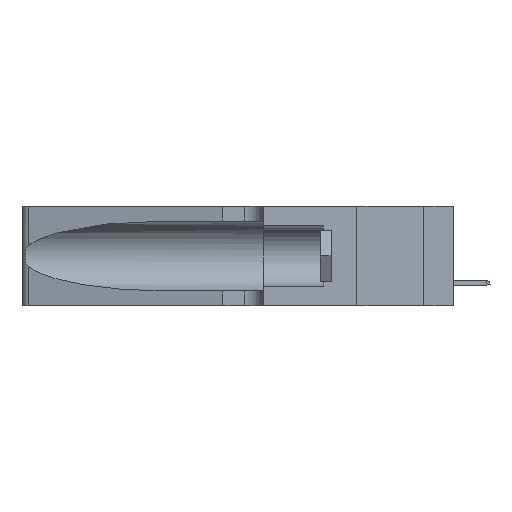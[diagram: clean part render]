
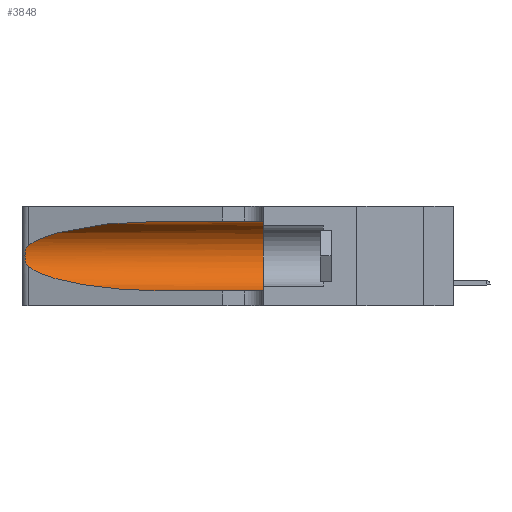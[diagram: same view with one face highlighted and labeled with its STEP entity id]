
A CAD part, left-side view. The second image highlights one B-rep face of the part: STEP entity #3848.
In plain terms, the highlighted cylindrical face has radius 3.308 mm (diameter 6.617 mm), a partial arc.
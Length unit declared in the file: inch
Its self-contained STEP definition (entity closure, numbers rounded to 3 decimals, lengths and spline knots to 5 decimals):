
#426 = EDGE_CURVE ( 'NONE', #11697, #22639, #37055, .T. ) ;
#994 = CARTESIAN_POINT ( 'NONE',  ( 0.25639, 1.23186, 0.15144 ) ) ;
#1021 = ORIENTED_EDGE ( 'NONE', *, *, #30124, .F. ) ;
#1545 = EDGE_CURVE ( 'NONE', #43997, #11697, #33295, .T. ) ;
#1990 = CARTESIAN_POINT ( 'NONE',  ( 0.25854, 1.2359, 0.20912 ) ) ;
#3632 = ORIENTED_EDGE ( 'NONE', *, *, #47640, .T. ) ;
#3848 = ADVANCED_FACE ( 'NONE', ( #8337 ), #12750, .F. ) ;
#4104 = CARTESIAN_POINT ( 'NONE',  ( 0.18966, 0.96281, 0.31525 ) ) ;
#4293 = CARTESIAN_POINT ( 'NONE',  ( 0.1305, 0.35, 0.05475 ) ) ;
#4942 =( BOUNDED_CURVE ( )  B_SPLINE_CURVE ( 3, ( #20145, #4104, #19639, #46591 ),
 .UNSPECIFIED., .F., .F. ) 
 B_SPLINE_CURVE_WITH_KNOTS ( ( 4, 4 ),
 ( 1.5708, 2.84003 ),
 .UNSPECIFIED. ) 
 CURVE ( )  GEOMETRIC_REPRESENTATION_ITEM ( )  RATIONAL_B_SPLINE_CURVE ( ( 1., 0.87, 0.87, 1. ) ) 
 REPRESENTATION_ITEM ( '' )  );
#5125 = CARTESIAN_POINT ( 'NONE',  ( 0.25487, 1.22718, 0.22369 ) ) ;
#5158 = CARTESIAN_POINT ( 'NONE',  ( 0.26018, 1.23835, 0.19895 ) ) ;
#5634 = CARTESIAN_POINT ( 'NONE',  ( 0.25555, 1.22994, 0.2215 ) ) ;
#5789 = CARTESIAN_POINT ( 'NONE',  ( 0.2373, 1.15595, 0.08982 ) ) ;
#6092 = CARTESIAN_POINT ( 'NONE',  ( 0.1305, 0.72297, 0.05475 ) ) ;
#6539 = VECTOR ( 'NONE', #46669, 39.37008 ) ;
#8337 = FACE_OUTER_BOUND ( 'NONE', #47398, .T. ) ;
#8387 = LINE ( 'NONE', #46920, #6539 ) ;
#8390 = CARTESIAN_POINT ( 'NONE',  ( 0.25856, 1.23593, 0.16098 ) ) ;
#11547 = VERTEX_POINT ( 'NONE', #5125 ) ;
#11697 = VERTEX_POINT ( 'NONE', #6092 ) ;
#12750 = CYLINDRICAL_SURFACE ( 'NONE', #36567, 0.13025 ) ;
#12976 = ORIENTED_EDGE ( 'NONE', *, *, #41182, .F. ) ;
#16011 = CARTESIAN_POINT ( 'NONE',  ( 0.25555, 1.22993, 0.14849 ) ) ;
#17529 = VERTEX_POINT ( 'NONE', #19064 ) ;
#19064 = CARTESIAN_POINT ( 'NONE',  ( 0.1305, 0.72297, 0.31525 ) ) ;
#19639 = CARTESIAN_POINT ( 'NONE',  ( 0.2373, 1.15595, 0.28018 ) ) ;
#20145 = CARTESIAN_POINT ( 'NONE',  ( 0.1305, 0.72297, 0.31525 ) ) ;
#21461 = B_SPLINE_CURVE_WITH_KNOTS ( 'NONE', 3,
 ( #28131, #5634, #39008, #35774, #1990, #5158, #30818, #45921, #42231, #8390, #34775, #994, #16011, #31064 ),
 .UNSPECIFIED., .F., .F.,
 ( 4, 2, 2, 2, 2, 2, 4 ),
 ( 0., 0.00027, 0.00053, 0.00107, 0.0016, 0.00187, 0.00214 ),
 .UNSPECIFIED. ) ;
#22549 = CARTESIAN_POINT ( 'NONE',  ( 0.18966, 0.96281, 0.05475 ) ) ;
#22639 = VERTEX_POINT ( 'NONE', #4293 ) ;
#23770 = DIRECTION ( 'NONE',  ( 0., 0., 1. ) ) ;
#23881 = AXIS2_PLACEMENT_3D ( 'NONE', #24027, #46276, #23770 ) ;
#24027 = CARTESIAN_POINT ( 'NONE',  ( 0.1305, 0.35, 0.185 ) ) ;
#24569 = CARTESIAN_POINT ( 'NONE',  ( 0.25487, 1.22718, 0.14631 ) ) ;
#26194 = DIRECTION ( 'NONE',  ( 0., -1., 0. ) ) ;
#27600 = DIRECTION ( 'NONE',  ( 0., -1., 0. ) ) ;
#28053 = EDGE_CURVE ( 'NONE', #17529, #11547, #4942, .T. ) ;
#28131 = CARTESIAN_POINT ( 'NONE',  ( 0.25487, 1.22718, 0.22369 ) ) ;
#29328 = VECTOR ( 'NONE', #26194, 39.37008 ) ;
#30124 = EDGE_CURVE ( 'NONE', #17529, #39484, #8387, .T. ) ;
#30818 = CARTESIAN_POINT ( 'NONE',  ( 0.26075, 1.23896, 0.19203 ) ) ;
#30935 = CIRCLE ( 'NONE', #23881, 0.13025 ) ;
#31064 = CARTESIAN_POINT ( 'NONE',  ( 0.25487, 1.22718, 0.14631 ) ) ;
#33295 =( BOUNDED_CURVE ( )  B_SPLINE_CURVE ( 3, ( #24569, #5789, #22549, #37129 ),
 .UNSPECIFIED., .F., .F. ) 
 B_SPLINE_CURVE_WITH_KNOTS ( ( 4, 4 ),
 ( 3.44316, 4.71239 ),
 .UNSPECIFIED. ) 
 CURVE ( )  GEOMETRIC_REPRESENTATION_ITEM ( )  RATIONAL_B_SPLINE_CURVE ( ( 1., 0.87, 0.87, 1. ) ) 
 REPRESENTATION_ITEM ( '' )  );
#33809 = CARTESIAN_POINT ( 'NONE',  ( 0.1305, 1.61858, 0.05475 ) ) ;
#34775 = CARTESIAN_POINT ( 'NONE',  ( 0.25789, 1.23486, 0.15765 ) ) ;
#35006 = ORIENTED_EDGE ( 'NONE', *, *, #28053, .T. ) ;
#35021 = ORIENTED_EDGE ( 'NONE', *, *, #1545, .T. ) ;
#35774 = CARTESIAN_POINT ( 'NONE',  ( 0.25787, 1.23484, 0.2124 ) ) ;
#36567 = AXIS2_PLACEMENT_3D ( 'NONE', #38219, #27600, #38465 ) ;
#37055 = LINE ( 'NONE', #33809, #29328 ) ;
#37129 = CARTESIAN_POINT ( 'NONE',  ( 0.1305, 0.72297, 0.05475 ) ) ;
#38219 = CARTESIAN_POINT ( 'NONE',  ( 0.1305, 1.61858, 0.185 ) ) ;
#38247 = CARTESIAN_POINT ( 'NONE',  ( 0.1305, 0.35, 0.31525 ) ) ;
#38465 = DIRECTION ( 'NONE',  ( 0., 0., -1. ) ) ;
#39008 = CARTESIAN_POINT ( 'NONE',  ( 0.25639, 1.23184, 0.21858 ) ) ;
#39484 = VERTEX_POINT ( 'NONE', #38247 ) ;
#40387 = CARTESIAN_POINT ( 'NONE',  ( 0.25487, 1.22718, 0.14631 ) ) ;
#41182 = EDGE_CURVE ( 'NONE', #39484, #22639, #30935, .T. ) ;
#41371 = ORIENTED_EDGE ( 'NONE', *, *, #426, .T. ) ;
#42231 = CARTESIAN_POINT ( 'NONE',  ( 0.26017, 1.23833, 0.17102 ) ) ;
#43997 = VERTEX_POINT ( 'NONE', #40387 ) ;
#45921 = CARTESIAN_POINT ( 'NONE',  ( 0.26075, 1.23896, 0.178 ) ) ;
#46276 = DIRECTION ( 'NONE',  ( 0., 1., 0. ) ) ;
#46591 = CARTESIAN_POINT ( 'NONE',  ( 0.25487, 1.22718, 0.22369 ) ) ;
#46669 = DIRECTION ( 'NONE',  ( 0., -1., 0. ) ) ;
#46920 = CARTESIAN_POINT ( 'NONE',  ( 0.1305, 1.61858, 0.31525 ) ) ;
#47398 = EDGE_LOOP ( 'NONE', ( #35006, #3632, #35021, #41371, #12976, #1021 ) ) ;
#47640 = EDGE_CURVE ( 'NONE', #11547, #43997, #21461, .T. ) ;
